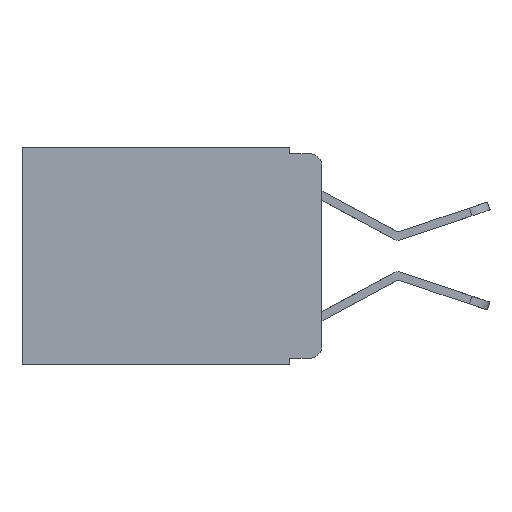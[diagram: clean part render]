
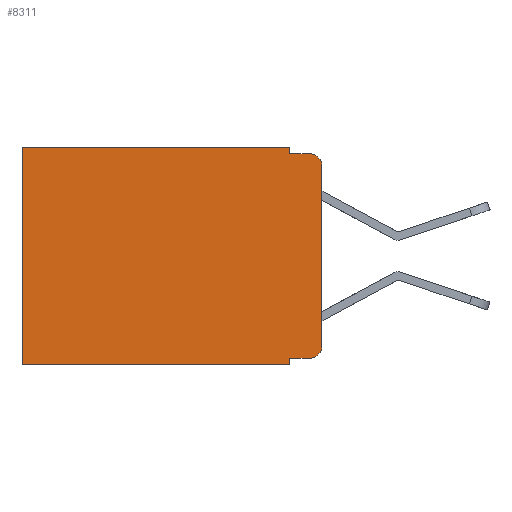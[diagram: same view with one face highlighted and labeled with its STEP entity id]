
A CAD part, left-side view. The second image highlights one B-rep face of the part: STEP entity #8311.
In plain terms, the highlighted planar face has unit normal (-1, 0, 0).
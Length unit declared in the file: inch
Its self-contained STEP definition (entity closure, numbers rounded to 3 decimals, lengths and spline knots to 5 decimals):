
#111 = EDGE_CURVE ( 'NONE', #15765, #15800, #16680, .T. ) ;
#366 = DIRECTION ( 'NONE',  ( 0., -1., 0. ) ) ;
#474 = VERTEX_POINT ( 'NONE', #16925 ) ;
#670 = CARTESIAN_POINT ( 'NONE',  ( 0.298, 0., -0.343 ) ) ;
#943 = CARTESIAN_POINT ( 'NONE',  ( 0.298, 0.02, -0.03 ) ) ;
#1045 = VERTEX_POINT ( 'NONE', #7236 ) ;
#1082 = EDGE_CURVE ( 'NONE', #1045, #17628, #10374, .T. ) ;
#1319 = CARTESIAN_POINT ( 'NONE',  ( 0.298, 0.473, -0.343 ) ) ;
#1577 = ORIENTED_EDGE ( 'NONE', *, *, #4720, .F. ) ;
#1981 = LINE ( 'NONE', #3417, #17147 ) ;
#2024 = VECTOR ( 'NONE', #9007, 39.37008 ) ;
#2251 = ORIENTED_EDGE ( 'NONE', *, *, #17290, .F. ) ;
#2261 = ORIENTED_EDGE ( 'NONE', *, *, #7249, .T. ) ;
#2682 = VECTOR ( 'NONE', #17327, 39.37008 ) ;
#3208 = VERTEX_POINT ( 'NONE', #3266 ) ;
#3266 = CARTESIAN_POINT ( 'NONE',  ( 0.298, 0., -0.03 ) ) ;
#3403 = CARTESIAN_POINT ( 'NONE',  ( 0.298, 0., 0. ) ) ;
#3417 = CARTESIAN_POINT ( 'NONE',  ( 0.298, 0.051, -0.333 ) ) ;
#3541 = LINE ( 'NONE', #9284, #2024 ) ;
#3770 = LINE ( 'NONE', #13412, #9502 ) ;
#4672 = VERTEX_POINT ( 'NONE', #8678 ) ;
#4720 = EDGE_CURVE ( 'NONE', #13005, #1045, #9292, .T. ) ;
#4849 = ORIENTED_EDGE ( 'NONE', *, *, #111, .F. ) ;
#4860 = CARTESIAN_POINT ( 'NONE',  ( 0.298, 0.02, -0.01 ) ) ;
#4942 = FACE_OUTER_BOUND ( 'NONE', #12525, .T. ) ;
#5375 = CARTESIAN_POINT ( 'NONE',  ( 0.298, 0.051, 0. ) ) ;
#5719 = CARTESIAN_POINT ( 'NONE',  ( 0.298, 0.02, -0.313 ) ) ;
#5954 = CARTESIAN_POINT ( 'NONE',  ( 0.298, 0.051, 0. ) ) ;
#6312 = AXIS2_PLACEMENT_3D ( 'NONE', #943, #6416, #17335 ) ;
#6416 = DIRECTION ( 'NONE',  ( -1., 0., 0. ) ) ;
#6540 = LINE ( 'NONE', #5375, #8293 ) ;
#6620 = DIRECTION ( 'NONE',  ( 0., 0., -1. ) ) ;
#7236 = CARTESIAN_POINT ( 'NONE',  ( 0.298, 0.051, -0.343 ) ) ;
#7249 = EDGE_CURVE ( 'NONE', #474, #17628, #3770, .T. ) ;
#7278 = CARTESIAN_POINT ( 'NONE',  ( 0.298, 0.051, -0.01 ) ) ;
#7456 = DIRECTION ( 'NONE',  ( 0., -1., 0. ) ) ;
#7627 = VECTOR ( 'NONE', #16902, 39.37008 ) ;
#8024 = AXIS2_PLACEMENT_3D ( 'NONE', #5719, #8330, #11275 ) ;
#8293 = VECTOR ( 'NONE', #17293, 39.37008 ) ;
#8311 = ADVANCED_FACE ( 'NONE', ( #4942 ), #13155, .F. ) ;
#8330 = DIRECTION ( 'NONE',  ( -1., 0., 0. ) ) ;
#8372 = ORIENTED_EDGE ( 'NONE', *, *, #14553, .T. ) ;
#8678 = CARTESIAN_POINT ( 'NONE',  ( 0.298, 0.02, -0.333 ) ) ;
#8968 = DIRECTION ( 'NONE',  ( 1., 0., 0. ) ) ;
#9007 = DIRECTION ( 'NONE',  ( 0., 0., -1. ) ) ;
#9284 = CARTESIAN_POINT ( 'NONE',  ( 0.298, 0., 0. ) ) ;
#9292 = LINE ( 'NONE', #17247, #2682 ) ;
#9502 = VECTOR ( 'NONE', #6620, 39.37008 ) ;
#10097 = ORIENTED_EDGE ( 'NONE', *, *, #14661, .F. ) ;
#10374 = LINE ( 'NONE', #670, #7627 ) ;
#10667 = CARTESIAN_POINT ( 'NONE',  ( 0.298, 0., -0.313 ) ) ;
#11130 = VECTOR ( 'NONE', #366, 39.37008 ) ;
#11275 = DIRECTION ( 'NONE',  ( 0., 0., -1. ) ) ;
#11654 = DIRECTION ( 'NONE',  ( 0., 1., 0. ) ) ;
#12129 = CARTESIAN_POINT ( 'NONE',  ( 0.298, 0.051, -0.333 ) ) ;
#12525 = EDGE_LOOP ( 'NONE', ( #2251, #16147, #4849, #10097, #13271, #2261, #12939, #1577, #8372, #14719 ) ) ;
#12604 = VERTEX_POINT ( 'NONE', #5954 ) ;
#12939 = ORIENTED_EDGE ( 'NONE', *, *, #1082, .F. ) ;
#12990 = CARTESIAN_POINT ( 'NONE',  ( 0.298, 0., 0. ) ) ;
#13005 = VERTEX_POINT ( 'NONE', #12129 ) ;
#13155 = PLANE ( 'NONE',  #13742 ) ;
#13271 = ORIENTED_EDGE ( 'NONE', *, *, #14532, .T. ) ;
#13412 = CARTESIAN_POINT ( 'NONE',  ( 0.298, 0.473, 0. ) ) ;
#13742 = AXIS2_PLACEMENT_3D ( 'NONE', #3403, #8968, #14412 ) ;
#14345 = CIRCLE ( 'NONE', #8024, 0.02 ) ;
#14412 = DIRECTION ( 'NONE',  ( 0., 0., -1. ) ) ;
#14532 = EDGE_CURVE ( 'NONE', #12604, #474, #17029, .T. ) ;
#14553 = EDGE_CURVE ( 'NONE', #13005, #4672, #1981, .T. ) ;
#14661 = EDGE_CURVE ( 'NONE', #12604, #15765, #6540, .T. ) ;
#14719 = ORIENTED_EDGE ( 'NONE', *, *, #16517, .T. ) ;
#15072 = VERTEX_POINT ( 'NONE', #10667 ) ;
#15765 = VERTEX_POINT ( 'NONE', #17218 ) ;
#15800 = VERTEX_POINT ( 'NONE', #4860 ) ;
#16005 = VECTOR ( 'NONE', #11654, 39.37008 ) ;
#16147 = ORIENTED_EDGE ( 'NONE', *, *, #16919, .T. ) ;
#16517 = EDGE_CURVE ( 'NONE', #4672, #15072, #14345, .T. ) ;
#16606 = CIRCLE ( 'NONE', #6312, 0.02 ) ;
#16680 = LINE ( 'NONE', #7278, #11130 ) ;
#16902 = DIRECTION ( 'NONE',  ( 0., 1., 0. ) ) ;
#16919 = EDGE_CURVE ( 'NONE', #3208, #15800, #16606, .T. ) ;
#16925 = CARTESIAN_POINT ( 'NONE',  ( 0.298, 0.473, 0. ) ) ;
#17029 = LINE ( 'NONE', #12990, #16005 ) ;
#17147 = VECTOR ( 'NONE', #7456, 39.37008 ) ;
#17218 = CARTESIAN_POINT ( 'NONE',  ( 0.298, 0.051, -0.01 ) ) ;
#17247 = CARTESIAN_POINT ( 'NONE',  ( 0.298, 0.051, 0. ) ) ;
#17290 = EDGE_CURVE ( 'NONE', #3208, #15072, #3541, .T. ) ;
#17293 = DIRECTION ( 'NONE',  ( 0., 0., -1. ) ) ;
#17327 = DIRECTION ( 'NONE',  ( 0., 0., -1. ) ) ;
#17335 = DIRECTION ( 'NONE',  ( 0., 0., -1. ) ) ;
#17628 = VERTEX_POINT ( 'NONE', #1319 ) ;
